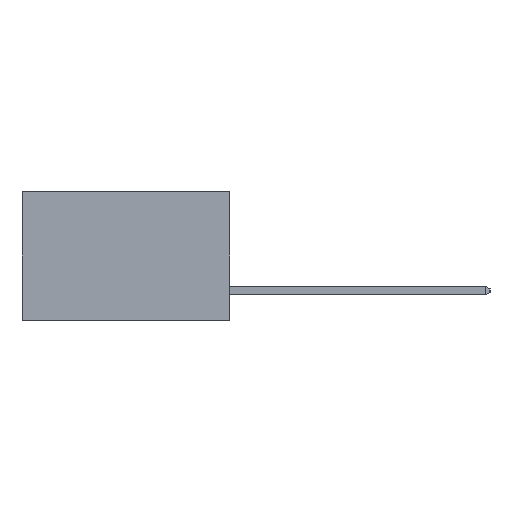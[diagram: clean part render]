
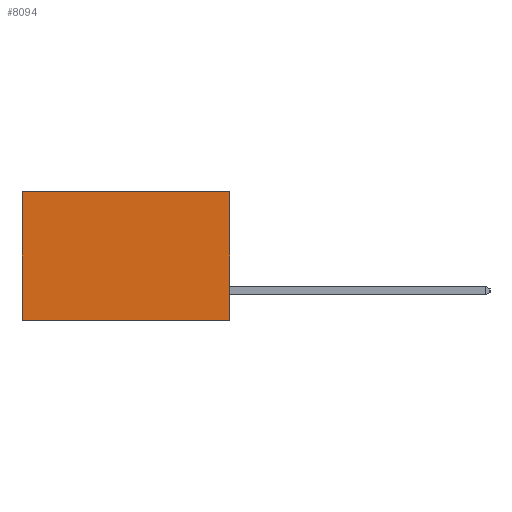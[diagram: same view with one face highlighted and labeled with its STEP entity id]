
A CAD part, left-side view. The second image highlights one B-rep face of the part: STEP entity #8094.
In plain terms, the highlighted planar face has unit normal (-1, 0, 0).
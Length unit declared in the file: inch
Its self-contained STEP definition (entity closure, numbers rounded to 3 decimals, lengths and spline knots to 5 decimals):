
#600 = VERTEX_POINT ( 'NONE', #13097 ) ;
#776 = CARTESIAN_POINT ( 'NONE',  ( 0.298, 0., -0.37 ) ) ;
#2753 = EDGE_LOOP ( 'NONE', ( #10467, #10831, #5285, #17821 ) ) ;
#3952 = LINE ( 'NONE', #18589, #12074 ) ;
#4028 = EDGE_CURVE ( 'NONE', #600, #14514, #11272, .T. ) ;
#4195 = CARTESIAN_POINT ( 'NONE',  ( 0.298, 0., 0. ) ) ;
#4199 = VECTOR ( 'NONE', #9436, 39.37008 ) ;
#4418 = CARTESIAN_POINT ( 'NONE',  ( 0.298, 0.6, -0.37 ) ) ;
#4658 = AXIS2_PLACEMENT_3D ( 'NONE', #10629, #20360, #14335 ) ;
#5285 = ORIENTED_EDGE ( 'NONE', *, *, #14385, .F. ) ;
#7094 = DIRECTION ( 'NONE',  ( 0., 1., 0. ) ) ;
#8094 = ADVANCED_FACE ( 'NONE', ( #14719 ), #10988, .F. ) ;
#8529 = VERTEX_POINT ( 'NONE', #776 ) ;
#9030 = CARTESIAN_POINT ( 'NONE',  ( 0.298, 0.6, 0. ) ) ;
#9155 = DIRECTION ( 'NONE',  ( 0., 0., -1. ) ) ;
#9174 = EDGE_CURVE ( 'NONE', #15247, #600, #21072, .T. ) ;
#9436 = DIRECTION ( 'NONE',  ( 0., 1., 0. ) ) ;
#9509 = CARTESIAN_POINT ( 'NONE',  ( 0.298, 0., 0. ) ) ;
#9820 = VECTOR ( 'NONE', #13971, 39.37008 ) ;
#10467 = ORIENTED_EDGE ( 'NONE', *, *, #4028, .T. ) ;
#10629 = CARTESIAN_POINT ( 'NONE',  ( 0.298, 0., 0. ) ) ;
#10831 = ORIENTED_EDGE ( 'NONE', *, *, #19143, .F. ) ;
#10988 = PLANE ( 'NONE',  #4658 ) ;
#11272 = LINE ( 'NONE', #9030, #20013 ) ;
#12074 = VECTOR ( 'NONE', #7094, 39.37008 ) ;
#13097 = CARTESIAN_POINT ( 'NONE',  ( 0.298, 0.6, 0. ) ) ;
#13971 = DIRECTION ( 'NONE',  ( 0., 0., -1. ) ) ;
#14335 = DIRECTION ( 'NONE',  ( 0., 0., -1. ) ) ;
#14385 = EDGE_CURVE ( 'NONE', #15247, #8529, #18062, .T. ) ;
#14514 = VERTEX_POINT ( 'NONE', #4418 ) ;
#14719 = FACE_OUTER_BOUND ( 'NONE', #2753, .T. ) ;
#15247 = VERTEX_POINT ( 'NONE', #17692 ) ;
#17692 = CARTESIAN_POINT ( 'NONE',  ( 0.298, 0., 0. ) ) ;
#17821 = ORIENTED_EDGE ( 'NONE', *, *, #9174, .T. ) ;
#18062 = LINE ( 'NONE', #4195, #9820 ) ;
#18589 = CARTESIAN_POINT ( 'NONE',  ( 0.298, 0., -0.37 ) ) ;
#19143 = EDGE_CURVE ( 'NONE', #8529, #14514, #3952, .T. ) ;
#20013 = VECTOR ( 'NONE', #9155, 39.37008 ) ;
#20360 = DIRECTION ( 'NONE',  ( 1., 0., 0. ) ) ;
#21072 = LINE ( 'NONE', #9509, #4199 ) ;
